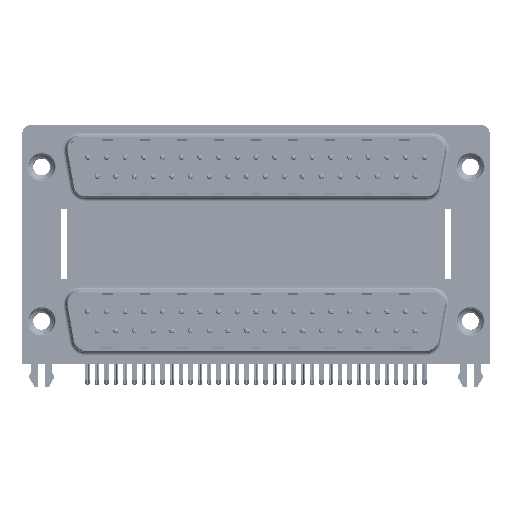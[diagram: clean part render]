
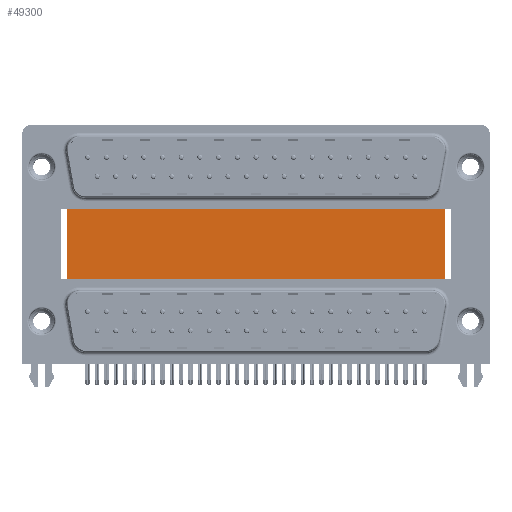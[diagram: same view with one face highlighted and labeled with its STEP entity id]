
A CAD part, top view. The second image highlights one B-rep face of the part: STEP entity #49300.
In plain terms, the highlighted planar face has unit normal (0, 0, 1).
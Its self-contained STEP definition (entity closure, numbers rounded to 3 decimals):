
#757 = CARTESIAN_POINT ( 'NONE',  ( 59.71, -3.735, -12. ) ) ;
#1797 = LINE ( 'NONE', #22892, #42702 ) ;
#5809 = VECTOR ( 'NONE', #12061, 1000. ) ;
#7710 = VERTEX_POINT ( 'NONE', #36773 ) ;
#9272 = ORIENTED_EDGE ( 'NONE', *, *, #27946, .T. ) ;
#12061 = DIRECTION ( 'NONE',  ( 1., 0., 0. ) ) ;
#17930 = EDGE_LOOP ( 'NONE', ( #39604, #52262, #39499, #9272 ) ) ;
#19272 = CARTESIAN_POINT ( 'NONE',  ( 59.71, 16.585, -12. ) ) ;
#19872 = DIRECTION ( 'NONE',  ( -1., 0., 0. ) ) ;
#20173 = CARTESIAN_POINT ( 'NONE',  ( 3.79, -3.735, -12. ) ) ;
#22412 = VECTOR ( 'NONE', #49745, 1000. ) ;
#22892 = CARTESIAN_POINT ( 'NONE',  ( 3.79, 16.585, -12. ) ) ;
#27946 = EDGE_CURVE ( 'NONE', #7710, #31604, #1797, .T. ) ;
#28660 = CARTESIAN_POINT ( 'NONE',  ( 3.79, 16.585, -12. ) ) ;
#28810 = FACE_OUTER_BOUND ( 'NONE', #17930, .T. ) ;
#31251 = EDGE_CURVE ( 'NONE', #31604, #50470, #40437, .T. ) ;
#31604 = VERTEX_POINT ( 'NONE', #52849 ) ;
#33253 = LINE ( 'NONE', #28660, #47008 ) ;
#33508 = CARTESIAN_POINT ( 'NONE',  ( 59.71, 16.585, -12. ) ) ;
#35226 = EDGE_CURVE ( 'NONE', #35817, #50470, #45955, .T. ) ;
#35817 = VERTEX_POINT ( 'NONE', #19272 ) ;
#36773 = CARTESIAN_POINT ( 'NONE',  ( 3.79, 16.585, -12. ) ) ;
#39381 = DIRECTION ( 'NONE',  ( 0., -1., 0. ) ) ;
#39499 = ORIENTED_EDGE ( 'NONE', *, *, #50372, .F. ) ;
#39604 = ORIENTED_EDGE ( 'NONE', *, *, #31251, .T. ) ;
#40437 = LINE ( 'NONE', #20173, #5809 ) ;
#40972 = CARTESIAN_POINT ( 'NONE',  ( 3.79, 16.585, -12. ) ) ;
#42702 = VECTOR ( 'NONE', #39381, 1000. ) ;
#44490 = PLANE ( 'NONE',  #45241 ) ;
#45241 = AXIS2_PLACEMENT_3D ( 'NONE', #40972, #49088, #19872 ) ;
#45955 = LINE ( 'NONE', #33508, #22412 ) ;
#45958 = DIRECTION ( 'NONE',  ( 1., 0., 0. ) ) ;
#47008 = VECTOR ( 'NONE', #45958, 1000. ) ;
#49088 = DIRECTION ( 'NONE',  ( 0., 0., -1. ) ) ;
#49300 = ADVANCED_FACE ( 'NONE', ( #28810 ), #44490, .F. ) ;
#49745 = DIRECTION ( 'NONE',  ( 0., -1., 0. ) ) ;
#50372 = EDGE_CURVE ( 'NONE', #7710, #35817, #33253, .T. ) ;
#50470 = VERTEX_POINT ( 'NONE', #757 ) ;
#52262 = ORIENTED_EDGE ( 'NONE', *, *, #35226, .F. ) ;
#52849 = CARTESIAN_POINT ( 'NONE',  ( 3.79, -3.735, -12. ) ) ;
